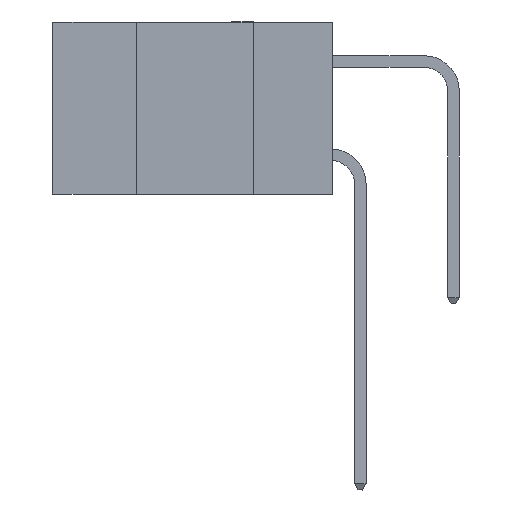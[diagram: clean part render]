
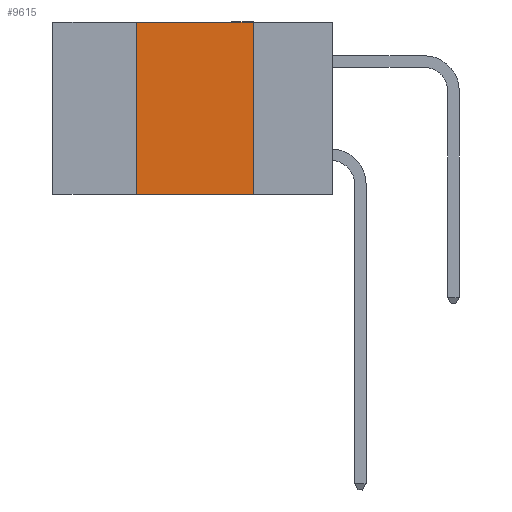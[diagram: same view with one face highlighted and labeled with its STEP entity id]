
A CAD part, left-side view. The second image highlights one B-rep face of the part: STEP entity #9615.
In plain terms, the highlighted planar face has unit normal (-1, 0, 0).
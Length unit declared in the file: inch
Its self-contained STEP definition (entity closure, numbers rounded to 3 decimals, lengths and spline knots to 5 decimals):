
#283 = ORIENTED_EDGE ( 'NONE', *, *, #8472, .F. ) ;
#714 = VERTEX_POINT ( 'NONE', #11194 ) ;
#733 = VECTOR ( 'NONE', #13801, 39.37008 ) ;
#772 = ORIENTED_EDGE ( 'NONE', *, *, #4814, .F. ) ;
#775 = VECTOR ( 'NONE', #1555, 39.37008 ) ;
#849 = VECTOR ( 'NONE', #9957, 39.37008 ) ;
#917 = LINE ( 'NONE', #7616, #733 ) ;
#1154 = VERTEX_POINT ( 'NONE', #5559 ) ;
#1555 = DIRECTION ( 'NONE',  ( 0., -1., 0. ) ) ;
#1898 = EDGE_LOOP ( 'NONE', ( #772, #283, #8714, #10811 ) ) ;
#2172 = VECTOR ( 'NONE', #6539, 39.37008 ) ;
#4157 = LINE ( 'NONE', #14308, #775 ) ;
#4237 = LINE ( 'NONE', #7365, #849 ) ;
#4673 = FACE_OUTER_BOUND ( 'NONE', #1898, .T. ) ;
#4814 = EDGE_CURVE ( 'NONE', #15794, #714, #4237, .T. ) ;
#5029 = CARTESIAN_POINT ( 'NONE',  ( 0., 0.42, -0.37 ) ) ;
#5074 = CARTESIAN_POINT ( 'NONE',  ( 0., 0.6, 0. ) ) ;
#5559 = CARTESIAN_POINT ( 'NONE',  ( 0., 0.42, 0. ) ) ;
#6235 = PLANE ( 'NONE',  #9126 ) ;
#6240 = CARTESIAN_POINT ( 'NONE',  ( 0., 0.17, 0. ) ) ;
#6539 = DIRECTION ( 'NONE',  ( 0., 0., 1. ) ) ;
#7365 = CARTESIAN_POINT ( 'NONE',  ( 0., 0.17, 0. ) ) ;
#7561 = DIRECTION ( 'NONE',  ( 0., 0., -1. ) ) ;
#7564 = EDGE_CURVE ( 'NONE', #8608, #1154, #12804, .T. ) ;
#7614 = DIRECTION ( 'NONE',  ( 1., 0., 0. ) ) ;
#7616 = CARTESIAN_POINT ( 'NONE',  ( 0., 0.6, 0. ) ) ;
#8472 = EDGE_CURVE ( 'NONE', #1154, #15794, #917, .T. ) ;
#8608 = VERTEX_POINT ( 'NONE', #5029 ) ;
#8714 = ORIENTED_EDGE ( 'NONE', *, *, #7564, .F. ) ;
#9079 = CARTESIAN_POINT ( 'NONE',  ( 0., 0.42, 0. ) ) ;
#9126 = AXIS2_PLACEMENT_3D ( 'NONE', #5074, #7614, #7561 ) ;
#9615 = ADVANCED_FACE ( 'NONE', ( #4673 ), #6235, .F. ) ;
#9957 = DIRECTION ( 'NONE',  ( 0., 0., -1. ) ) ;
#10811 = ORIENTED_EDGE ( 'NONE', *, *, #13010, .T. ) ;
#11194 = CARTESIAN_POINT ( 'NONE',  ( 0., 0.17, -0.37 ) ) ;
#12804 = LINE ( 'NONE', #9079, #2172 ) ;
#13010 = EDGE_CURVE ( 'NONE', #8608, #714, #4157, .T. ) ;
#13801 = DIRECTION ( 'NONE',  ( 0., -1., 0. ) ) ;
#14308 = CARTESIAN_POINT ( 'NONE',  ( 0., 0.6, -0.37 ) ) ;
#15794 = VERTEX_POINT ( 'NONE', #6240 ) ;
